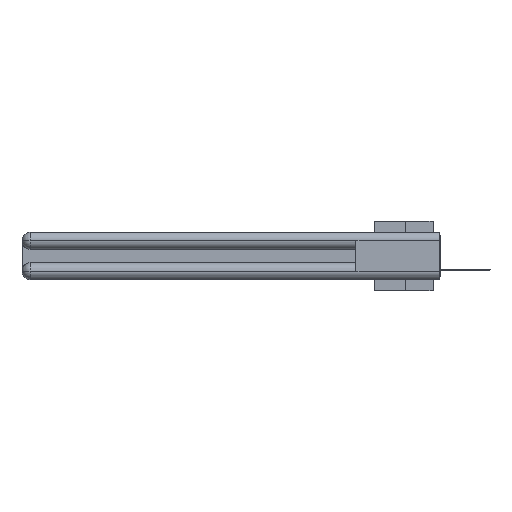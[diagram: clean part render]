
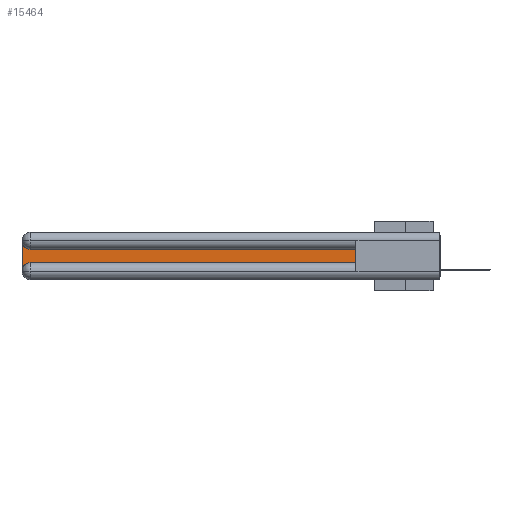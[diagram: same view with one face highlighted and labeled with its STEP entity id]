
A CAD part, left-side view. The second image highlights one B-rep face of the part: STEP entity #15464.
In plain terms, the highlighted planar face has unit normal (-1, 0, 0).
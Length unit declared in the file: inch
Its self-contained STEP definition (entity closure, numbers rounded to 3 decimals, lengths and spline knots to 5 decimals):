
#337 = VECTOR ( 'NONE', #31693, 39.37008 ) ;
#360 = CIRCLE ( 'NONE', #22562, 0.06 ) ;
#582 = LINE ( 'NONE', #12890, #30742 ) ;
#649 = ORIENTED_EDGE ( 'NONE', *, *, #3341, .T. ) ;
#1811 = DIRECTION ( 'NONE',  ( 1., 0., 0. ) ) ;
#1854 = EDGE_CURVE ( 'NONE', #16885, #25256, #22477, .T. ) ;
#2763 = ORIENTED_EDGE ( 'NONE', *, *, #19278, .T. ) ;
#2879 = CARTESIAN_POINT ( 'NONE',  ( 0.075, 0.6, -0.1225 ) ) ;
#3341 = EDGE_CURVE ( 'NONE', #25256, #5295, #14323, .T. ) ;
#3782 = CARTESIAN_POINT ( 'NONE',  ( 0.075, 2.94, -0.2775 ) ) ;
#5172 = DIRECTION ( 'NONE',  ( 0., 0., -1. ) ) ;
#5295 = VERTEX_POINT ( 'NONE', #18475 ) ;
#5781 = EDGE_LOOP ( 'NONE', ( #27550, #20574, #12842, #27637, #649, #2763 ) ) ;
#5898 = DIRECTION ( 'NONE',  ( 0., 0., -1. ) ) ;
#9092 = DIRECTION ( 'NONE',  ( 0., 0., -1. ) ) ;
#10425 = LINE ( 'NONE', #25287, #12741 ) ;
#11404 = DIRECTION ( 'NONE',  ( 0., -1., 0. ) ) ;
#12128 = PLANE ( 'NONE',  #28015 ) ;
#12741 = VECTOR ( 'NONE', #5898, 39.37008 ) ;
#12842 = ORIENTED_EDGE ( 'NONE', *, *, #20957, .T. ) ;
#12890 = CARTESIAN_POINT ( 'NONE',  ( 0.075, 0.6, -0.2175 ) ) ;
#13076 = CARTESIAN_POINT ( 'NONE',  ( 0.075, 3., -0.2775 ) ) ;
#14323 = LINE ( 'NONE', #24174, #24441 ) ;
#14702 = LINE ( 'NONE', #2879, #337 ) ;
#15260 = CARTESIAN_POINT ( 'NONE',  ( 0.075, 2.94, -0.2175 ) ) ;
#15464 = ADVANCED_FACE ( 'NONE', ( #22277 ), #12128, .F. ) ;
#16118 = DIRECTION ( 'NONE',  ( 0., 0., -1. ) ) ;
#16282 = AXIS2_PLACEMENT_3D ( 'NONE', #3782, #1811, #9092 ) ;
#16885 = VERTEX_POINT ( 'NONE', #13076 ) ;
#17288 = DIRECTION ( 'NONE',  ( 1., 0., 0. ) ) ;
#18475 = CARTESIAN_POINT ( 'NONE',  ( 0.075, 0.6, -0.2175 ) ) ;
#18685 = VERTEX_POINT ( 'NONE', #25042 ) ;
#19278 = EDGE_CURVE ( 'NONE', #5295, #18685, #582, .T. ) ;
#20574 = ORIENTED_EDGE ( 'NONE', *, *, #31010, .T. ) ;
#20957 = EDGE_CURVE ( 'NONE', #23155, #16885, #10425, .T. ) ;
#21936 = VERTEX_POINT ( 'NONE', #23936 ) ;
#22277 = FACE_OUTER_BOUND ( 'NONE', #5781, .T. ) ;
#22477 = CIRCLE ( 'NONE', #16282, 0.06 ) ;
#22562 = AXIS2_PLACEMENT_3D ( 'NONE', #30548, #28278, #16118 ) ;
#23155 = VERTEX_POINT ( 'NONE', #28495 ) ;
#23936 = CARTESIAN_POINT ( 'NONE',  ( 0.075, 2.94, -0.1225 ) ) ;
#24174 = CARTESIAN_POINT ( 'NONE',  ( 0.075, 0.6, -0.2175 ) ) ;
#24441 = VECTOR ( 'NONE', #11404, 39.37008 ) ;
#25042 = CARTESIAN_POINT ( 'NONE',  ( 0.075, 0.6, -0.1225 ) ) ;
#25256 = VERTEX_POINT ( 'NONE', #15260 ) ;
#25287 = CARTESIAN_POINT ( 'NONE',  ( 0.075, 3., -0.2175 ) ) ;
#27550 = ORIENTED_EDGE ( 'NONE', *, *, #29143, .T. ) ;
#27637 = ORIENTED_EDGE ( 'NONE', *, *, #1854, .T. ) ;
#27765 = DIRECTION ( 'NONE',  ( 0., 0., 1. ) ) ;
#28015 = AXIS2_PLACEMENT_3D ( 'NONE', #31874, #17288, #5172 ) ;
#28278 = DIRECTION ( 'NONE',  ( 1., 0., 0. ) ) ;
#28495 = CARTESIAN_POINT ( 'NONE',  ( 0.075, 3., -0.0625 ) ) ;
#29143 = EDGE_CURVE ( 'NONE', #18685, #21936, #14702, .T. ) ;
#30548 = CARTESIAN_POINT ( 'NONE',  ( 0.075, 2.94, -0.0625 ) ) ;
#30742 = VECTOR ( 'NONE', #27765, 39.37008 ) ;
#31010 = EDGE_CURVE ( 'NONE', #21936, #23155, #360, .T. ) ;
#31693 = DIRECTION ( 'NONE',  ( 0., 1., 0. ) ) ;
#31874 = CARTESIAN_POINT ( 'NONE',  ( 0.075, 3., -0.1225 ) ) ;
